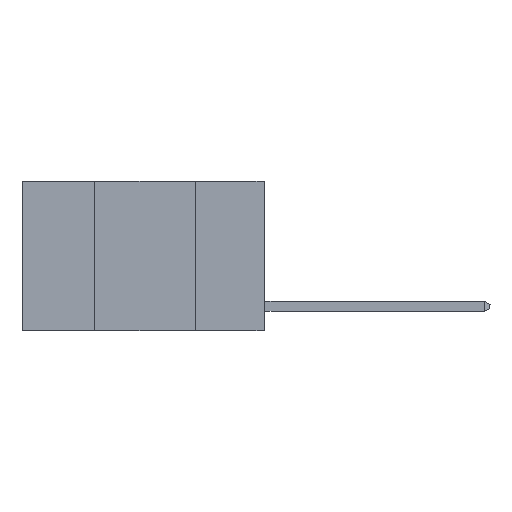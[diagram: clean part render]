
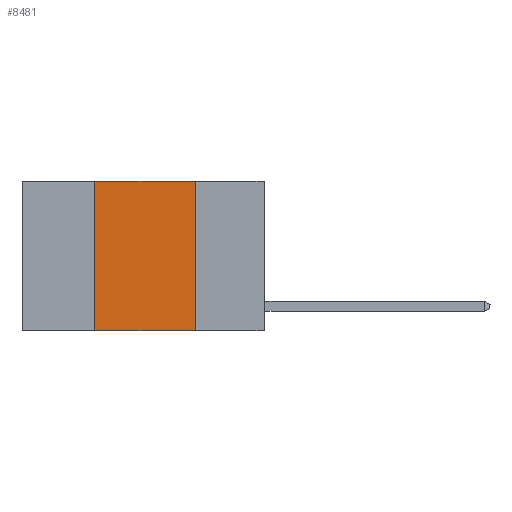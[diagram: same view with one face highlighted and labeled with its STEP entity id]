
A CAD part, left-side view. The second image highlights one B-rep face of the part: STEP entity #8481.
In plain terms, the highlighted planar face has unit normal (-1, 0, 0).
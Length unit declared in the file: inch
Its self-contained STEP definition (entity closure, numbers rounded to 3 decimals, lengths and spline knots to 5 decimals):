
#625 = CARTESIAN_POINT ( 'NONE',  ( 0., 0.42, -0.37 ) ) ;
#738 = DIRECTION ( 'NONE',  ( 1., 0., 0. ) ) ;
#887 = LINE ( 'NONE', #17731, #9216 ) ;
#1149 = EDGE_CURVE ( 'NONE', #11752, #17771, #1870, .T. ) ;
#1870 = LINE ( 'NONE', #17864, #5746 ) ;
#3124 = VERTEX_POINT ( 'NONE', #625 ) ;
#4879 = EDGE_CURVE ( 'NONE', #16553, #11752, #9840, .T. ) ;
#5308 = EDGE_CURVE ( 'NONE', #3124, #16553, #13705, .T. ) ;
#5746 = VECTOR ( 'NONE', #19555, 39.37008 ) ;
#5767 = FACE_OUTER_BOUND ( 'NONE', #15399, .T. ) ;
#5894 = AXIS2_PLACEMENT_3D ( 'NONE', #10694, #738, #12345 ) ;
#8240 = ORIENTED_EDGE ( 'NONE', *, *, #4879, .F. ) ;
#8323 = CARTESIAN_POINT ( 'NONE',  ( 0., 0.17, 0. ) ) ;
#8481 = ADVANCED_FACE ( 'NONE', ( #5767 ), #20697, .F. ) ;
#8775 = DIRECTION ( 'NONE',  ( 0., -1., 0. ) ) ;
#9216 = VECTOR ( 'NONE', #19442, 39.37008 ) ;
#9840 = LINE ( 'NONE', #20444, #18167 ) ;
#10694 = CARTESIAN_POINT ( 'NONE',  ( 0., 0.6, 0. ) ) ;
#11222 = ORIENTED_EDGE ( 'NONE', *, *, #5308, .F. ) ;
#11321 = ORIENTED_EDGE ( 'NONE', *, *, #18734, .T. ) ;
#11752 = VERTEX_POINT ( 'NONE', #8323 ) ;
#12345 = DIRECTION ( 'NONE',  ( 0., 0., -1. ) ) ;
#13705 = LINE ( 'NONE', #16512, #18691 ) ;
#15399 = EDGE_LOOP ( 'NONE', ( #18996, #8240, #11222, #11321 ) ) ;
#16512 = CARTESIAN_POINT ( 'NONE',  ( 0., 0.42, 0. ) ) ;
#16553 = VERTEX_POINT ( 'NONE', #16684 ) ;
#16684 = CARTESIAN_POINT ( 'NONE',  ( 0., 0.42, 0. ) ) ;
#17731 = CARTESIAN_POINT ( 'NONE',  ( 0., 0.6, -0.37 ) ) ;
#17771 = VERTEX_POINT ( 'NONE', #18453 ) ;
#17864 = CARTESIAN_POINT ( 'NONE',  ( 0., 0.17, 0. ) ) ;
#18167 = VECTOR ( 'NONE', #8775, 39.37008 ) ;
#18453 = CARTESIAN_POINT ( 'NONE',  ( 0., 0.17, -0.37 ) ) ;
#18691 = VECTOR ( 'NONE', #21499, 39.37008 ) ;
#18734 = EDGE_CURVE ( 'NONE', #3124, #17771, #887, .T. ) ;
#18996 = ORIENTED_EDGE ( 'NONE', *, *, #1149, .F. ) ;
#19442 = DIRECTION ( 'NONE',  ( 0., -1., 0. ) ) ;
#19555 = DIRECTION ( 'NONE',  ( 0., 0., -1. ) ) ;
#20444 = CARTESIAN_POINT ( 'NONE',  ( 0., 0.6, 0. ) ) ;
#20697 = PLANE ( 'NONE',  #5894 ) ;
#21499 = DIRECTION ( 'NONE',  ( 0., 0., 1. ) ) ;
